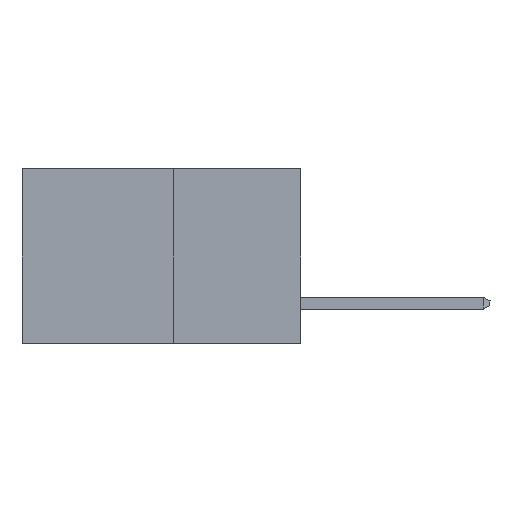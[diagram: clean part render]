
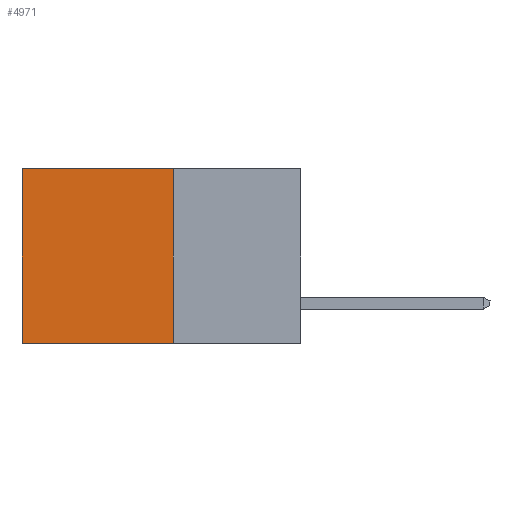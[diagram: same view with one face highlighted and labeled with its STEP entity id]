
A CAD part, left-side view. The second image highlights one B-rep face of the part: STEP entity #4971.
In plain terms, the highlighted planar face has unit normal (-1, 0, 0).
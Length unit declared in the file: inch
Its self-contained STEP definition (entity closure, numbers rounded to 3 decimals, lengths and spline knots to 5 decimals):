
#68 = DIRECTION ( 'NONE',  ( 0., 1., 0. ) ) ;
#219 = VECTOR ( 'NONE', #15376, 39.37008 ) ;
#451 = VECTOR ( 'NONE', #68, 39.37008 ) ;
#550 = CARTESIAN_POINT ( 'NONE',  ( 0.277, 0.59, -0.37 ) ) ;
#1231 = CARTESIAN_POINT ( 'NONE',  ( 0.277, 0.27, 0. ) ) ;
#2056 = VERTEX_POINT ( 'NONE', #550 ) ;
#3175 = AXIS2_PLACEMENT_3D ( 'NONE', #14572, #12053, #4793 ) ;
#3777 = LINE ( 'NONE', #1231, #451 ) ;
#4320 = LINE ( 'NONE', #14159, #219 ) ;
#4793 = DIRECTION ( 'NONE',  ( 0., 0., -1. ) ) ;
#4880 = PLANE ( 'NONE',  #3175 ) ;
#4971 = ADVANCED_FACE ( 'NONE', ( #12979 ), #4880, .F. ) ;
#5895 = ORIENTED_EDGE ( 'NONE', *, *, #11552, .F. ) ;
#6395 = CARTESIAN_POINT ( 'NONE',  ( 0.277, 0.59, -0.37 ) ) ;
#6474 = CARTESIAN_POINT ( 'NONE',  ( 0.277, 0.59, 0. ) ) ;
#7096 = VERTEX_POINT ( 'NONE', #7273 ) ;
#7273 = CARTESIAN_POINT ( 'NONE',  ( 0.277, 0.27, -0.37 ) ) ;
#7342 = CARTESIAN_POINT ( 'NONE',  ( 0.277, 0.27, 0. ) ) ;
#7435 = ORIENTED_EDGE ( 'NONE', *, *, #8789, .T. ) ;
#7555 = VERTEX_POINT ( 'NONE', #6474 ) ;
#7642 = LINE ( 'NONE', #6395, #8029 ) ;
#8029 = VECTOR ( 'NONE', #14972, 39.37008 ) ;
#8139 = CARTESIAN_POINT ( 'NONE',  ( 0.277, 0.27, -0.37 ) ) ;
#8789 = EDGE_CURVE ( 'NONE', #7555, #2056, #7642, .T. ) ;
#9110 = LINE ( 'NONE', #8139, #15223 ) ;
#9382 = EDGE_CURVE ( 'NONE', #9968, #7555, #3777, .T. ) ;
#9389 = DIRECTION ( 'NONE',  ( 0., 1., 0. ) ) ;
#9968 = VERTEX_POINT ( 'NONE', #7342 ) ;
#10865 = EDGE_LOOP ( 'NONE', ( #7435, #11886, #5895, #15256 ) ) ;
#11552 = EDGE_CURVE ( 'NONE', #9968, #7096, #4320, .T. ) ;
#11886 = ORIENTED_EDGE ( 'NONE', *, *, #13099, .F. ) ;
#12053 = DIRECTION ( 'NONE',  ( 1., 0., 0. ) ) ;
#12979 = FACE_OUTER_BOUND ( 'NONE', #10865, .T. ) ;
#13099 = EDGE_CURVE ( 'NONE', #7096, #2056, #9110, .T. ) ;
#14159 = CARTESIAN_POINT ( 'NONE',  ( 0.277, 0.27, -0.37 ) ) ;
#14572 = CARTESIAN_POINT ( 'NONE',  ( 0.277, 0.27, -0.37 ) ) ;
#14972 = DIRECTION ( 'NONE',  ( 0., 0., -1. ) ) ;
#15223 = VECTOR ( 'NONE', #9389, 39.37008 ) ;
#15256 = ORIENTED_EDGE ( 'NONE', *, *, #9382, .T. ) ;
#15376 = DIRECTION ( 'NONE',  ( 0., 0., -1. ) ) ;
